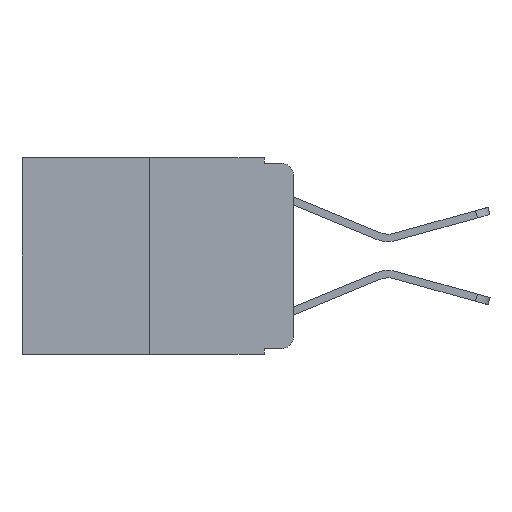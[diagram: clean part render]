
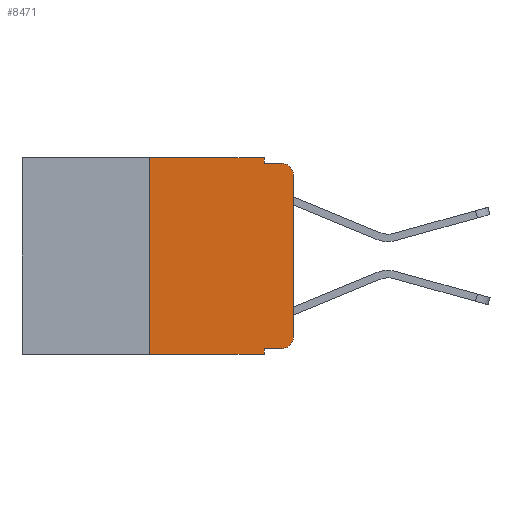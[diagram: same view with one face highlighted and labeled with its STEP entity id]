
A CAD part, left-side view. The second image highlights one B-rep face of the part: STEP entity #8471.
In plain terms, the highlighted planar face has unit normal (-1, 0, 0).
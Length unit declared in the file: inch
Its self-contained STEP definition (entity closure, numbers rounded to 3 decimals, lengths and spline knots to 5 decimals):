
#374 = ORIENTED_EDGE ( 'NONE', *, *, #2902, .T. ) ;
#618 = VECTOR ( 'NONE', #4364, 39.37008 ) ;
#694 = DIRECTION ( 'NONE',  ( 0., 0., -1. ) ) ;
#713 = DIRECTION ( 'NONE',  ( 0., 0., 1. ) ) ;
#919 = FACE_OUTER_BOUND ( 'NONE', #5898, .T. ) ;
#1006 = DIRECTION ( 'NONE',  ( 0., 0., -1. ) ) ;
#1486 = VERTEX_POINT ( 'NONE', #18949 ) ;
#2370 = CARTESIAN_POINT ( 'NONE',  ( 0., 0.473, -0.343 ) ) ;
#2796 = VECTOR ( 'NONE', #694, 39.37008 ) ;
#2806 = CARTESIAN_POINT ( 'NONE',  ( 0., 0.473, 0. ) ) ;
#2902 = EDGE_CURVE ( 'NONE', #16297, #18192, #5426, .T. ) ;
#3214 = LINE ( 'NONE', #2806, #618 ) ;
#3607 = ORIENTED_EDGE ( 'NONE', *, *, #6093, .T. ) ;
#3807 = EDGE_CURVE ( 'NONE', #14595, #12381, #12170, .T. ) ;
#3827 = CARTESIAN_POINT ( 'NONE',  ( 0., 0.02, -0.03 ) ) ;
#4131 = LINE ( 'NONE', #4577, #8365 ) ;
#4364 = DIRECTION ( 'NONE',  ( 0., -1., 0. ) ) ;
#4503 = CARTESIAN_POINT ( 'NONE',  ( 0., 0., -0.313 ) ) ;
#4515 = CARTESIAN_POINT ( 'NONE',  ( 0., 0.02, -0.313 ) ) ;
#4577 = CARTESIAN_POINT ( 'NONE',  ( 0., 0.051, -0.333 ) ) ;
#5426 = CIRCLE ( 'NONE', #10334, 0.02 ) ;
#5440 = CARTESIAN_POINT ( 'NONE',  ( 0., 0.051, -0.343 ) ) ;
#5898 = EDGE_LOOP ( 'NONE', ( #3607, #374, #13750, #18820, #10776, #18874, #14155, #13029, #8554, #18104 ) ) ;
#6093 = EDGE_CURVE ( 'NONE', #14904, #16297, #10163, .T. ) ;
#6108 = CARTESIAN_POINT ( 'NONE',  ( 0., 0.02, -0.01 ) ) ;
#6145 = VECTOR ( 'NONE', #713, 39.37008 ) ;
#6222 = CARTESIAN_POINT ( 'NONE',  ( 0., 0.473, 0. ) ) ;
#6411 = PLANE ( 'NONE',  #12606 ) ;
#7695 = LINE ( 'NONE', #10012, #18996 ) ;
#7730 = CIRCLE ( 'NONE', #9918, 0.02 ) ;
#8190 = VECTOR ( 'NONE', #13460, 39.37008 ) ;
#8233 = DIRECTION ( 'NONE',  ( 0., 0., -1. ) ) ;
#8365 = VECTOR ( 'NONE', #12251, 39.37008 ) ;
#8471 = ADVANCED_FACE ( 'NONE', ( #919 ), #6411, .F. ) ;
#8554 = ORIENTED_EDGE ( 'NONE', *, *, #12872, .T. ) ;
#9022 = CARTESIAN_POINT ( 'NONE',  ( 0., 0.25, 0. ) ) ;
#9042 = VECTOR ( 'NONE', #14700, 39.37008 ) ;
#9626 = EDGE_CURVE ( 'NONE', #17407, #18192, #14226, .T. ) ;
#9918 = AXIS2_PLACEMENT_3D ( 'NONE', #4515, #13881, #16656 ) ;
#9926 = CARTESIAN_POINT ( 'NONE',  ( 0., 0.25, -0.343 ) ) ;
#9958 = DIRECTION ( 'NONE',  ( -1., 0., 0. ) ) ;
#10012 = CARTESIAN_POINT ( 'NONE',  ( 0., 0.051, 0. ) ) ;
#10163 = LINE ( 'NONE', #18251, #6145 ) ;
#10334 = AXIS2_PLACEMENT_3D ( 'NONE', #3827, #9958, #8233 ) ;
#10776 = ORIENTED_EDGE ( 'NONE', *, *, #16372, .F. ) ;
#11103 = CARTESIAN_POINT ( 'NONE',  ( 0., 0.25, 0. ) ) ;
#11354 = EDGE_CURVE ( 'NONE', #1486, #14904, #7730, .T. ) ;
#11528 = EDGE_CURVE ( 'NONE', #12483, #17407, #13363, .T. ) ;
#11891 = EDGE_CURVE ( 'NONE', #13435, #15086, #7695, .T. ) ;
#11957 = DIRECTION ( 'NONE',  ( 0., -1., 0. ) ) ;
#12170 = LINE ( 'NONE', #9022, #8190 ) ;
#12241 = DIRECTION ( 'NONE',  ( 0., 0., -1. ) ) ;
#12251 = DIRECTION ( 'NONE',  ( 0., -1., 0. ) ) ;
#12312 = LINE ( 'NONE', #2370, #9042 ) ;
#12381 = VERTEX_POINT ( 'NONE', #11103 ) ;
#12483 = VERTEX_POINT ( 'NONE', #17180 ) ;
#12606 = AXIS2_PLACEMENT_3D ( 'NONE', #6222, #16719, #12241 ) ;
#12872 = EDGE_CURVE ( 'NONE', #13435, #1486, #4131, .T. ) ;
#13029 = ORIENTED_EDGE ( 'NONE', *, *, #11891, .F. ) ;
#13363 = LINE ( 'NONE', #18690, #2796 ) ;
#13435 = VERTEX_POINT ( 'NONE', #16013 ) ;
#13460 = DIRECTION ( 'NONE',  ( 0., 0., 1. ) ) ;
#13750 = ORIENTED_EDGE ( 'NONE', *, *, #9626, .F. ) ;
#13881 = DIRECTION ( 'NONE',  ( -1., 0., 0. ) ) ;
#14155 = ORIENTED_EDGE ( 'NONE', *, *, #17385, .T. ) ;
#14226 = LINE ( 'NONE', #16421, #17776 ) ;
#14595 = VERTEX_POINT ( 'NONE', #9926 ) ;
#14700 = DIRECTION ( 'NONE',  ( 0., -1., 0. ) ) ;
#14904 = VERTEX_POINT ( 'NONE', #4503 ) ;
#15086 = VERTEX_POINT ( 'NONE', #5440 ) ;
#16013 = CARTESIAN_POINT ( 'NONE',  ( 0., 0.051, -0.333 ) ) ;
#16297 = VERTEX_POINT ( 'NONE', #19358 ) ;
#16372 = EDGE_CURVE ( 'NONE', #12381, #12483, #3214, .T. ) ;
#16421 = CARTESIAN_POINT ( 'NONE',  ( 0., 0.051, -0.01 ) ) ;
#16656 = DIRECTION ( 'NONE',  ( 0., 0., -1. ) ) ;
#16719 = DIRECTION ( 'NONE',  ( 1., 0., 0. ) ) ;
#17180 = CARTESIAN_POINT ( 'NONE',  ( 0., 0.051, 0. ) ) ;
#17385 = EDGE_CURVE ( 'NONE', #14595, #15086, #12312, .T. ) ;
#17407 = VERTEX_POINT ( 'NONE', #18913 ) ;
#17776 = VECTOR ( 'NONE', #11957, 39.37008 ) ;
#18104 = ORIENTED_EDGE ( 'NONE', *, *, #11354, .T. ) ;
#18192 = VERTEX_POINT ( 'NONE', #6108 ) ;
#18251 = CARTESIAN_POINT ( 'NONE',  ( 0., 0., 0. ) ) ;
#18690 = CARTESIAN_POINT ( 'NONE',  ( 0., 0.051, 0. ) ) ;
#18820 = ORIENTED_EDGE ( 'NONE', *, *, #11528, .F. ) ;
#18874 = ORIENTED_EDGE ( 'NONE', *, *, #3807, .F. ) ;
#18913 = CARTESIAN_POINT ( 'NONE',  ( 0., 0.051, -0.01 ) ) ;
#18949 = CARTESIAN_POINT ( 'NONE',  ( 0., 0.02, -0.333 ) ) ;
#18996 = VECTOR ( 'NONE', #1006, 39.37008 ) ;
#19358 = CARTESIAN_POINT ( 'NONE',  ( 0., 0., -0.03 ) ) ;
